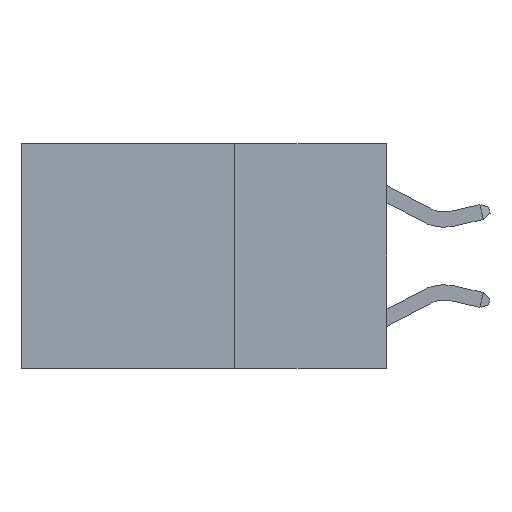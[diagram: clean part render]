
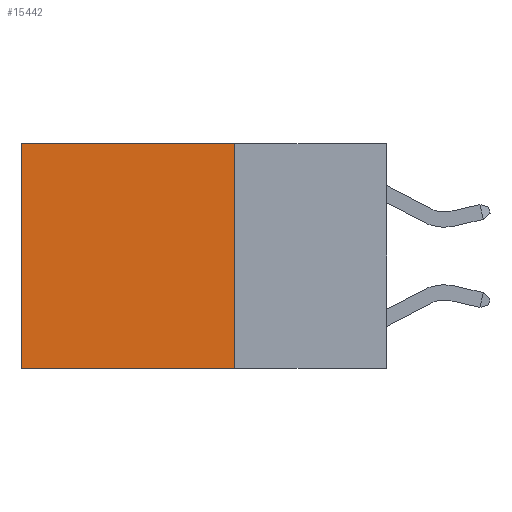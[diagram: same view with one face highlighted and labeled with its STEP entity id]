
A CAD part, left-side view. The second image highlights one B-rep face of the part: STEP entity #15442.
In plain terms, the highlighted planar face has unit normal (-1, 0, 0).
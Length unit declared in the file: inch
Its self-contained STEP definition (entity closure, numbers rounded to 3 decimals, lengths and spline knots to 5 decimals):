
#121 = VECTOR ( 'NONE', #16456, 39.37008 ) ;
#211 = EDGE_CURVE ( 'NONE', #1109, #18272, #613, .T. ) ;
#241 = FACE_OUTER_BOUND ( 'NONE', #6482, .T. ) ;
#613 = LINE ( 'NONE', #18423, #121 ) ;
#902 = VECTOR ( 'NONE', #18817, 39.37008 ) ;
#1054 = DIRECTION ( 'NONE',  ( 1., 0., 0. ) ) ;
#1109 = VERTEX_POINT ( 'NONE', #8769 ) ;
#1725 = LINE ( 'NONE', #10928, #17153 ) ;
#2176 = ORIENTED_EDGE ( 'NONE', *, *, #4845, .T. ) ;
#2719 = DIRECTION ( 'NONE',  ( 0., 0., -1. ) ) ;
#4195 = CARTESIAN_POINT ( 'NONE',  ( 0.2625, 0.6, 0. ) ) ;
#4845 = EDGE_CURVE ( 'NONE', #18272, #15770, #11784, .T. ) ;
#5668 = CARTESIAN_POINT ( 'NONE',  ( 0.2625, 0.25, 0. ) ) ;
#5895 = EDGE_CURVE ( 'NONE', #7959, #15770, #8973, .T. ) ;
#6482 = EDGE_LOOP ( 'NONE', ( #2176, #11310, #16807, #8373 ) ) ;
#7189 = PLANE ( 'NONE',  #15557 ) ;
#7854 = VECTOR ( 'NONE', #2719, 39.37008 ) ;
#7959 = VERTEX_POINT ( 'NONE', #8060 ) ;
#8060 = CARTESIAN_POINT ( 'NONE',  ( 0.2625, 0.25, -0.37 ) ) ;
#8373 = ORIENTED_EDGE ( 'NONE', *, *, #211, .T. ) ;
#8769 = CARTESIAN_POINT ( 'NONE',  ( 0.2625, 0.25, 0. ) ) ;
#8973 = LINE ( 'NONE', #12857, #902 ) ;
#10821 = CARTESIAN_POINT ( 'NONE',  ( 0.2625, 0.6, -0.37 ) ) ;
#10928 = CARTESIAN_POINT ( 'NONE',  ( 0.2625, 0.25, 0. ) ) ;
#11310 = ORIENTED_EDGE ( 'NONE', *, *, #5895, .F. ) ;
#11784 = LINE ( 'NONE', #4195, #7854 ) ;
#12857 = CARTESIAN_POINT ( 'NONE',  ( 0.2625, 0.25, -0.37 ) ) ;
#14440 = EDGE_CURVE ( 'NONE', #1109, #7959, #1725, .T. ) ;
#15442 = ADVANCED_FACE ( 'NONE', ( #241 ), #7189, .F. ) ;
#15557 = AXIS2_PLACEMENT_3D ( 'NONE', #5668, #1054, #17522 ) ;
#15770 = VERTEX_POINT ( 'NONE', #10821 ) ;
#16456 = DIRECTION ( 'NONE',  ( 0., 1., 0. ) ) ;
#16807 = ORIENTED_EDGE ( 'NONE', *, *, #14440, .F. ) ;
#17153 = VECTOR ( 'NONE', #18342, 39.37008 ) ;
#17522 = DIRECTION ( 'NONE',  ( 0., 0., -1. ) ) ;
#18272 = VERTEX_POINT ( 'NONE', #19092 ) ;
#18342 = DIRECTION ( 'NONE',  ( 0., 0., -1. ) ) ;
#18423 = CARTESIAN_POINT ( 'NONE',  ( 0.2625, 0.25, 0. ) ) ;
#18817 = DIRECTION ( 'NONE',  ( 0., 1., 0. ) ) ;
#19092 = CARTESIAN_POINT ( 'NONE',  ( 0.2625, 0.6, 0. ) ) ;
